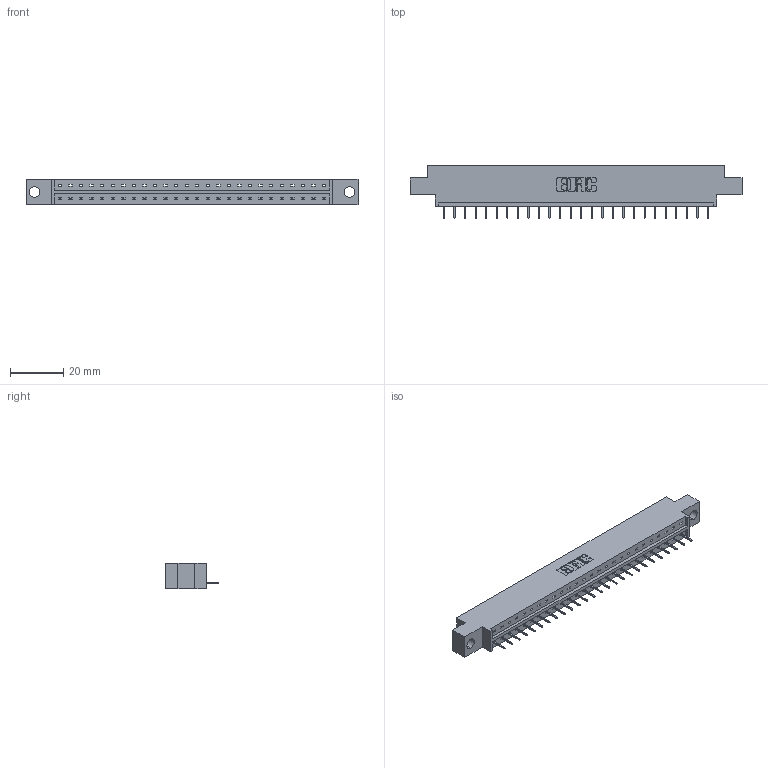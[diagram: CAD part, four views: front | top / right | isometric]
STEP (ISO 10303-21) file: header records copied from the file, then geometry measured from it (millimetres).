
FILE_DESCRIPTION (( 'STEP AP203' ), '1' );
FILE_NAME ('833-026-524-604.STEP', '2020-06-02T04:18:24', ( '' ), ( '' ), 'SwSTEP 2.0', 'SolidWorks 2020', '' );
FILE_SCHEMA (( 'CONFIG_CONTROL_DESIGN' ));
Length unit declared in the file: inch
Products named in the file (3): 833-026-524-604; 833 Part_Offset - .156 Dia - TH; 345-292-001_345-293-124
Assembly tree (27 placements, depth 2):
  833-026-524-604
    833 Part_Offset - .156 Dia - TH
    345-292-001_345-293-124  x26
Bounding box: 124.56 x 19.69 x 9.4 mm (x, y, z)
Volume: 11978.5 mm3; surface area: 12496.2 mm2
Topology: 27 solids, 27 shells, 1730 faces, 5003 edges, 3230 vertices
Faces by surface type: plane 1322, cylinder 408
Entity records: 18173 total; most frequent: CARTESIAN_POINT 3144, ORIENTED_EDGE 3106, DIRECTION 2685, EDGE_CURVE 1553, VECTOR 1429, LINE 1429, VERTEX_POINT 1030, AXIS2_PLACEMENT_3D 628
